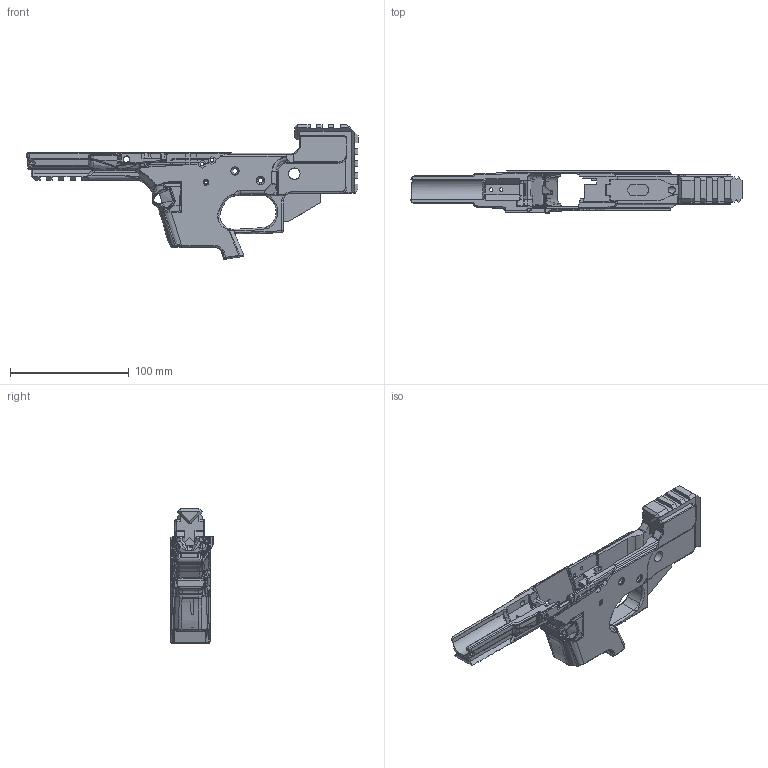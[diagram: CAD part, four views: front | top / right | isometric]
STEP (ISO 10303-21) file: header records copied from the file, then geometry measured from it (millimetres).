
FILE_DESCRIPTION(/* description */ (''),/* implementation_level */ '2;1');
FILE_NAME(/* name */ '3090_45_RAR_CLEAN v3.step',/* time_stamp */ '2022-09-15T14:33:44-05:00',/* author */ (''),/* organization */ (''),/* preprocessor_version */ 'ST-DEVELOPER v19',/* originating_system */ 'Autodesk Translation Framework v11.7.0.108',/* authorisation */ '');
FILE_SCHEMA (('AUTOMOTIVE_DESIGN { 1 0 10303 214 3 1 1 }'));
Products named in the file (1): 3090_45_RAR_CLEAN
Bounding box: 279.81 x 35.88 x 113.49 mm (x, y, z)
Volume: 185235 mm3; surface area: 70606.5 mm2
Topology: 1 solids, 1 shells, 1799 faces, 4889 edges, 3055 vertices
Faces by surface type: plane 656, bspline 648, cylinder 358, torus 82, cone 38, sphere 17
Full cylindrical faces by diameter (mm): 2 x1, 2.5 x2, 3 x6, 4.064 x4, 4.089 x1, 5.2 x2, 5.537 x1, 5.939 x4, 6.5 x3, 7.5 x1, 9.652 x2
Entity records: 99656 total; most frequent: CARTESIAN_POINT 59158, ORIENTED_EDGE 9712, DIRECTION 6742, EDGE_CURVE 4856, VERTEX_POINT 3055, AXIS2_PLACEMENT_3D 2335, LINE 2072, VECTOR 2072
